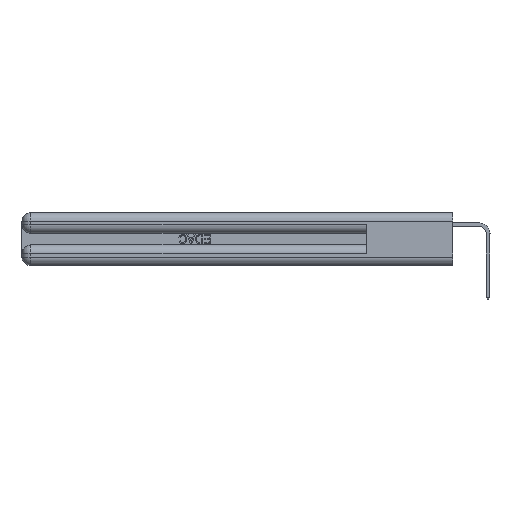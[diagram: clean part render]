
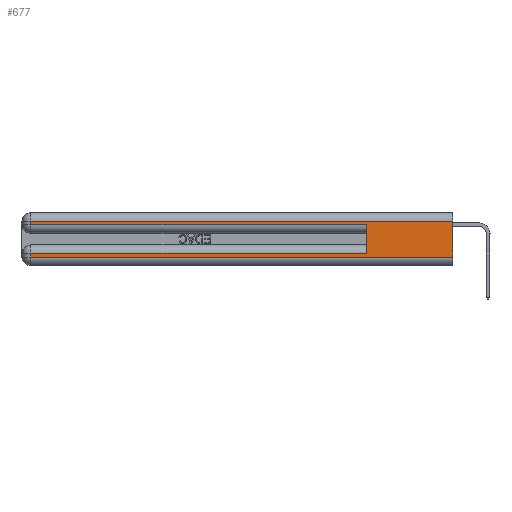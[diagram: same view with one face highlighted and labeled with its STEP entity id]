
A CAD part, left-side view. The second image highlights one B-rep face of the part: STEP entity #677.
In plain terms, the highlighted planar face has unit normal (-1, 0, 0).
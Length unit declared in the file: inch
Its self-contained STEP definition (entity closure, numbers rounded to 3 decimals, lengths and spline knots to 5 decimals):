
#677 = ADVANCED_FACE ( 'NONE', ( #41905 ), #45929, .F. ) ;
#3476 = LINE ( 'NONE', #25271, #42019 ) ;
#3541 = CARTESIAN_POINT ( 'NONE',  ( 0., 0., 0.31 ) ) ;
#3715 = ORIENTED_EDGE ( 'NONE', *, *, #6732, .F. ) ;
#3876 = DIRECTION ( 'NONE',  ( 1., 0., 0. ) ) ;
#4545 = VECTOR ( 'NONE', #16213, 39.37008 ) ;
#5020 = LINE ( 'NONE', #49697, #24266 ) ;
#5074 = EDGE_CURVE ( 'NONE', #21839, #14340, #15931, .T. ) ;
#5560 = VERTEX_POINT ( 'NONE', #15658 ) ;
#6732 = EDGE_CURVE ( 'NONE', #5560, #24308, #18856, .T. ) ;
#7336 = EDGE_CURVE ( 'NONE', #36908, #34439, #33268, .T. ) ;
#9028 = EDGE_CURVE ( 'NONE', #5560, #43844, #46817, .T. ) ;
#10367 = CARTESIAN_POINT ( 'NONE',  ( 0., 0., 0.085 ) ) ;
#10641 = EDGE_LOOP ( 'NONE', ( #11267, #18000, #33734, #39206, #3715, #30322, #15242, #40872 ) ) ;
#11267 = ORIENTED_EDGE ( 'NONE', *, *, #20128, .F. ) ;
#13760 = CARTESIAN_POINT ( 'NONE',  ( 0., 0., 0.06 ) ) ;
#14340 = VERTEX_POINT ( 'NONE', #13760 ) ;
#15242 = ORIENTED_EDGE ( 'NONE', *, *, #46855, .T. ) ;
#15658 = CARTESIAN_POINT ( 'NONE',  ( 0., 0.6, 0.085 ) ) ;
#15818 = LINE ( 'NONE', #32517, #24895 ) ;
#15931 = LINE ( 'NONE', #35468, #4545 ) ;
#16042 = VECTOR ( 'NONE', #37350, 39.37008 ) ;
#16213 = DIRECTION ( 'NONE',  ( 0., -1., 0. ) ) ;
#17394 = EDGE_CURVE ( 'NONE', #34439, #18503, #3476, .T. ) ;
#17691 = CARTESIAN_POINT ( 'NONE',  ( 0., 0., 0.31 ) ) ;
#18000 = ORIENTED_EDGE ( 'NONE', *, *, #7336, .T. ) ;
#18503 = VERTEX_POINT ( 'NONE', #39231 ) ;
#18856 = LINE ( 'NONE', #26462, #48390 ) ;
#18866 = CARTESIAN_POINT ( 'NONE',  ( 0., 2.94, 0.37 ) ) ;
#20128 = EDGE_CURVE ( 'NONE', #36908, #14340, #5020, .T. ) ;
#21374 = DIRECTION ( 'NONE',  ( 0., 0., -1. ) ) ;
#21839 = VERTEX_POINT ( 'NONE', #28315 ) ;
#23017 = VECTOR ( 'NONE', #45756, 39.37008 ) ;
#23025 = CARTESIAN_POINT ( 'NONE',  ( 0., 0., 0.37 ) ) ;
#24266 = VECTOR ( 'NONE', #30518, 39.37008 ) ;
#24308 = VERTEX_POINT ( 'NONE', #29424 ) ;
#24895 = VECTOR ( 'NONE', #36394, 39.37008 ) ;
#25271 = CARTESIAN_POINT ( 'NONE',  ( 0., 2.94, 0.37 ) ) ;
#26270 = CARTESIAN_POINT ( 'NONE',  ( 0., 2.94, 0.31 ) ) ;
#26462 = CARTESIAN_POINT ( 'NONE',  ( 0., 0.6, 0.145 ) ) ;
#26963 = LINE ( 'NONE', #18866, #28171 ) ;
#28171 = VECTOR ( 'NONE', #45819, 39.37008 ) ;
#28315 = CARTESIAN_POINT ( 'NONE',  ( 0., 2.94, 0.06 ) ) ;
#29424 = CARTESIAN_POINT ( 'NONE',  ( 0., 0.6, 0.285 ) ) ;
#30322 = ORIENTED_EDGE ( 'NONE', *, *, #9028, .T. ) ;
#30518 = DIRECTION ( 'NONE',  ( 0., 0., -1. ) ) ;
#30802 = DIRECTION ( 'NONE',  ( 0., 0., -1. ) ) ;
#31138 = CARTESIAN_POINT ( 'NONE',  ( 0., 2.94, 0.085 ) ) ;
#32517 = CARTESIAN_POINT ( 'NONE',  ( 0., 0., 0.285 ) ) ;
#33268 = LINE ( 'NONE', #3541, #23017 ) ;
#33734 = ORIENTED_EDGE ( 'NONE', *, *, #17394, .T. ) ;
#34224 = DIRECTION ( 'NONE',  ( 0., 0., 1. ) ) ;
#34439 = VERTEX_POINT ( 'NONE', #26270 ) ;
#35468 = CARTESIAN_POINT ( 'NONE',  ( 0., 0., 0.06 ) ) ;
#36394 = DIRECTION ( 'NONE',  ( 0., -1., 0. ) ) ;
#36908 = VERTEX_POINT ( 'NONE', #17691 ) ;
#37350 = DIRECTION ( 'NONE',  ( 0., 1., 0. ) ) ;
#39206 = ORIENTED_EDGE ( 'NONE', *, *, #41521, .T. ) ;
#39231 = CARTESIAN_POINT ( 'NONE',  ( 0., 2.94, 0.285 ) ) ;
#40872 = ORIENTED_EDGE ( 'NONE', *, *, #5074, .T. ) ;
#41521 = EDGE_CURVE ( 'NONE', #18503, #24308, #15818, .T. ) ;
#41905 = FACE_OUTER_BOUND ( 'NONE', #10641, .T. ) ;
#42019 = VECTOR ( 'NONE', #21374, 39.37008 ) ;
#43844 = VERTEX_POINT ( 'NONE', #31138 ) ;
#44800 = AXIS2_PLACEMENT_3D ( 'NONE', #23025, #3876, #30802 ) ;
#45756 = DIRECTION ( 'NONE',  ( 0., 1., 0. ) ) ;
#45819 = DIRECTION ( 'NONE',  ( 0., 0., -1. ) ) ;
#45929 = PLANE ( 'NONE',  #44800 ) ;
#46817 = LINE ( 'NONE', #10367, #16042 ) ;
#46855 = EDGE_CURVE ( 'NONE', #43844, #21839, #26963, .T. ) ;
#48390 = VECTOR ( 'NONE', #34224, 39.37008 ) ;
#49697 = CARTESIAN_POINT ( 'NONE',  ( 0., 0., 0.37 ) ) ;
